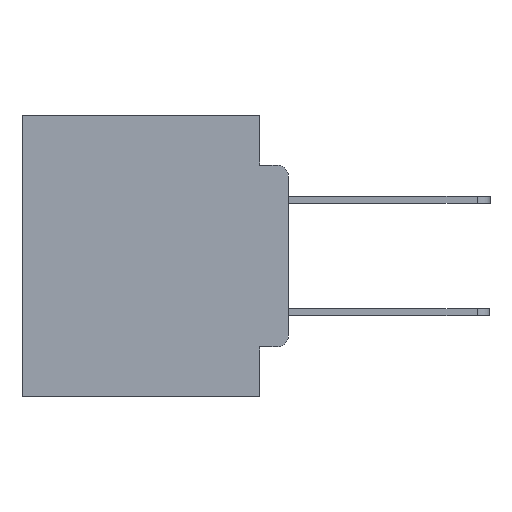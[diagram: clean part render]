
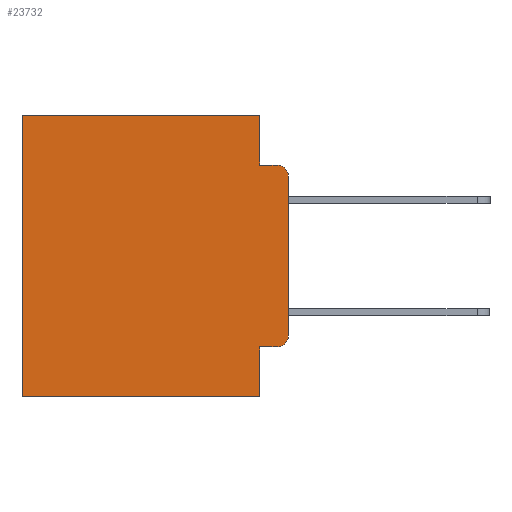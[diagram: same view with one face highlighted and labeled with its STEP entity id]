
A CAD part, left-side view. The second image highlights one B-rep face of the part: STEP entity #23732.
In plain terms, the highlighted planar face has unit normal (-1, 0, 0).
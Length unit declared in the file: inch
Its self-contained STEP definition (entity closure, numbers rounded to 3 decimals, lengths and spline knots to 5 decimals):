
#229 = LINE ( 'NONE', #19052, #22269 ) ;
#270 = VERTEX_POINT ( 'NONE', #10578 ) ;
#1227 = VERTEX_POINT ( 'NONE', #18007 ) ;
#2085 = CARTESIAN_POINT ( 'NONE',  ( 0.298, 0.02, -0.0885 ) ) ;
#2630 = FACE_OUTER_BOUND ( 'NONE', #7143, .T. ) ;
#2637 = EDGE_CURVE ( 'NONE', #26406, #25826, #22131, .T. ) ;
#2739 = VECTOR ( 'NONE', #26401, 39.37008 ) ;
#2985 = ORIENTED_EDGE ( 'NONE', *, *, #2637, .F. ) ;
#3945 = VECTOR ( 'NONE', #9633, 39.37008 ) ;
#4077 = EDGE_CURVE ( 'NONE', #7039, #25826, #14822, .T. ) ;
#4247 = VECTOR ( 'NONE', #25549, 39.37008 ) ;
#4401 = DIRECTION ( 'NONE',  ( 0., -1., 0. ) ) ;
#4841 = LINE ( 'NONE', #20602, #25919 ) ;
#5204 = VECTOR ( 'NONE', #4401, 39.37008 ) ;
#5499 = CARTESIAN_POINT ( 'NONE',  ( 0.298, 0.473, 0. ) ) ;
#5523 = CARTESIAN_POINT ( 'NONE',  ( 0.298, 0.473, -0.5 ) ) ;
#6077 = CARTESIAN_POINT ( 'NONE',  ( 0.298, 0.051, -0.0885 ) ) ;
#7039 = VERTEX_POINT ( 'NONE', #17401 ) ;
#7143 = EDGE_LOOP ( 'NONE', ( #23265, #17989, #2985, #13655, #22363, #16649, #14982, #24487, #10689, #13328 ) ) ;
#7399 = CARTESIAN_POINT ( 'NONE',  ( 0.298, 0.02, -0.3915 ) ) ;
#8043 = CARTESIAN_POINT ( 'NONE',  ( 0.298, 0.051, 0. ) ) ;
#8140 = DIRECTION ( 'NONE',  ( 0., 0., -1. ) ) ;
#8437 = LINE ( 'NONE', #24328, #2739 ) ;
#8481 = DIRECTION ( 'NONE',  ( 0., 1., 0. ) ) ;
#8903 = CARTESIAN_POINT ( 'NONE',  ( 0.298, 0.02, -0.1085 ) ) ;
#8961 = DIRECTION ( 'NONE',  ( -1., 0., 0. ) ) ;
#9577 = DIRECTION ( 'NONE',  ( 0., 0., -1. ) ) ;
#9633 = DIRECTION ( 'NONE',  ( 0., 1., 0. ) ) ;
#9815 = EDGE_CURVE ( 'NONE', #26976, #26406, #15569, .T. ) ;
#10578 = CARTESIAN_POINT ( 'NONE',  ( 0.298, 0., -0.3915 ) ) ;
#10689 = ORIENTED_EDGE ( 'NONE', *, *, #16908, .T. ) ;
#10812 = VERTEX_POINT ( 'NONE', #21419 ) ;
#11253 = EDGE_CURVE ( 'NONE', #10812, #1227, #4841, .T. ) ;
#11927 = VECTOR ( 'NONE', #21980, 39.37008 ) ;
#13328 = ORIENTED_EDGE ( 'NONE', *, *, #19752, .T. ) ;
#13509 = CARTESIAN_POINT ( 'NONE',  ( 0.298, 0.02, -0.4115 ) ) ;
#13655 = ORIENTED_EDGE ( 'NONE', *, *, #9815, .F. ) ;
#13706 = AXIS2_PLACEMENT_3D ( 'NONE', #8903, #8961, #26197 ) ;
#13893 = CARTESIAN_POINT ( 'NONE',  ( 0.298, 0., -0.5 ) ) ;
#14041 = EDGE_CURVE ( 'NONE', #1227, #19824, #15246, .T. ) ;
#14080 = EDGE_CURVE ( 'NONE', #14515, #19824, #25685, .T. ) ;
#14443 = PLANE ( 'NONE',  #19593 ) ;
#14515 = VERTEX_POINT ( 'NONE', #19693 ) ;
#14591 = EDGE_CURVE ( 'NONE', #7039, #270, #17549, .T. ) ;
#14822 = CIRCLE ( 'NONE', #13706, 0.02 ) ;
#14982 = ORIENTED_EDGE ( 'NONE', *, *, #14041, .F. ) ;
#15145 = CARTESIAN_POINT ( 'NONE',  ( 0.298, 0.051, 0. ) ) ;
#15246 = LINE ( 'NONE', #13893, #3945 ) ;
#15569 = LINE ( 'NONE', #15145, #4247 ) ;
#16649 = ORIENTED_EDGE ( 'NONE', *, *, #14080, .T. ) ;
#16806 = VERTEX_POINT ( 'NONE', #13509 ) ;
#16908 = EDGE_CURVE ( 'NONE', #10812, #16806, #8437, .T. ) ;
#17401 = CARTESIAN_POINT ( 'NONE',  ( 0.298, 0., -0.1085 ) ) ;
#17549 = LINE ( 'NONE', #17772, #11927 ) ;
#17772 = CARTESIAN_POINT ( 'NONE',  ( 0.298, 0., 0. ) ) ;
#17989 = ORIENTED_EDGE ( 'NONE', *, *, #4077, .T. ) ;
#18007 = CARTESIAN_POINT ( 'NONE',  ( 0.298, 0.051, -0.5 ) ) ;
#18259 = CARTESIAN_POINT ( 'NONE',  ( 0.298, 0.051, -0.0885 ) ) ;
#18592 = DIRECTION ( 'NONE',  ( 0., 0., -1. ) ) ;
#19052 = CARTESIAN_POINT ( 'NONE',  ( 0.298, 0., 0. ) ) ;
#19474 = CIRCLE ( 'NONE', #26749, 0.02 ) ;
#19560 = VECTOR ( 'NONE', #22454, 39.37008 ) ;
#19593 = AXIS2_PLACEMENT_3D ( 'NONE', #22812, #20831, #8140 ) ;
#19693 = CARTESIAN_POINT ( 'NONE',  ( 0.298, 0.473, 0. ) ) ;
#19752 = EDGE_CURVE ( 'NONE', #16806, #270, #19474, .T. ) ;
#19824 = VERTEX_POINT ( 'NONE', #5523 ) ;
#20602 = CARTESIAN_POINT ( 'NONE',  ( 0.298, 0.051, 0. ) ) ;
#20831 = DIRECTION ( 'NONE',  ( 1., 0., 0. ) ) ;
#21419 = CARTESIAN_POINT ( 'NONE',  ( 0.298, 0.051, -0.4115 ) ) ;
#21980 = DIRECTION ( 'NONE',  ( 0., 0., -1. ) ) ;
#22131 = LINE ( 'NONE', #18259, #5204 ) ;
#22213 = DIRECTION ( 'NONE',  ( -1., 0., 0. ) ) ;
#22269 = VECTOR ( 'NONE', #8481, 39.37008 ) ;
#22363 = ORIENTED_EDGE ( 'NONE', *, *, #25805, .T. ) ;
#22454 = DIRECTION ( 'NONE',  ( 0., 0., -1. ) ) ;
#22812 = CARTESIAN_POINT ( 'NONE',  ( 0.298, 0., 0. ) ) ;
#23265 = ORIENTED_EDGE ( 'NONE', *, *, #14591, .F. ) ;
#23732 = ADVANCED_FACE ( 'NONE', ( #2630 ), #14443, .F. ) ;
#24328 = CARTESIAN_POINT ( 'NONE',  ( 0.298, 0.051, -0.4115 ) ) ;
#24487 = ORIENTED_EDGE ( 'NONE', *, *, #11253, .F. ) ;
#25549 = DIRECTION ( 'NONE',  ( 0., 0., -1. ) ) ;
#25685 = LINE ( 'NONE', #5499, #19560 ) ;
#25805 = EDGE_CURVE ( 'NONE', #26976, #14515, #229, .T. ) ;
#25826 = VERTEX_POINT ( 'NONE', #2085 ) ;
#25919 = VECTOR ( 'NONE', #18592, 39.37008 ) ;
#26197 = DIRECTION ( 'NONE',  ( 0., 0., -1. ) ) ;
#26401 = DIRECTION ( 'NONE',  ( 0., -1., 0. ) ) ;
#26406 = VERTEX_POINT ( 'NONE', #6077 ) ;
#26749 = AXIS2_PLACEMENT_3D ( 'NONE', #7399, #22213, #9577 ) ;
#26976 = VERTEX_POINT ( 'NONE', #8043 ) ;
